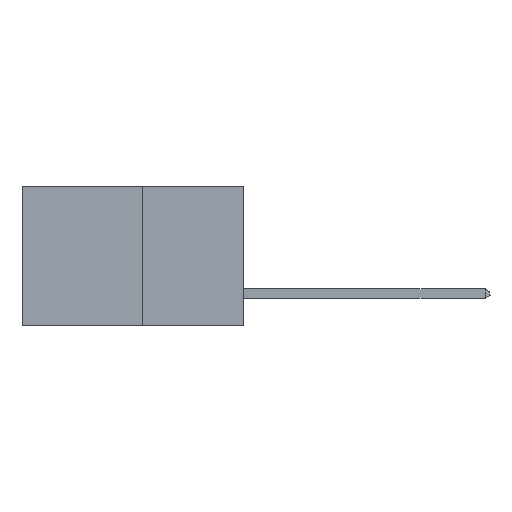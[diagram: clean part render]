
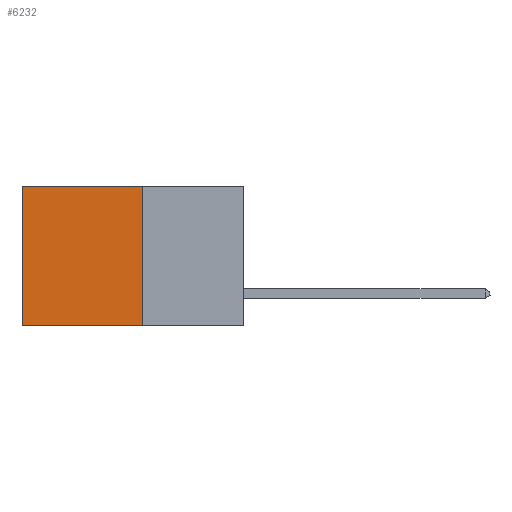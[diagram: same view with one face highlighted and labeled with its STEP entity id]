
A CAD part, left-side view. The second image highlights one B-rep face of the part: STEP entity #6232.
In plain terms, the highlighted planar face has unit normal (-1, 0, 0).
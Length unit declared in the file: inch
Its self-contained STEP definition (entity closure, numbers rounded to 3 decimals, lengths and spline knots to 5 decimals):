
#1770 = CARTESIAN_POINT ( 'NONE',  ( 0.277, 0.59, -0.37 ) ) ;
#2014 = LINE ( 'NONE', #5491, #26398 ) ;
#2191 = CARTESIAN_POINT ( 'NONE',  ( 0.277, 0.27, -0.37 ) ) ;
#2647 = CARTESIAN_POINT ( 'NONE',  ( 0.277, 0.27, 0. ) ) ;
#3800 = DIRECTION ( 'NONE',  ( 0., 0., -1. ) ) ;
#3831 = DIRECTION ( 'NONE',  ( 1., 0., 0. ) ) ;
#3864 = PLANE ( 'NONE',  #15335 ) ;
#4041 = CARTESIAN_POINT ( 'NONE',  ( 0.277, 0.27, -0.37 ) ) ;
#5218 = VERTEX_POINT ( 'NONE', #20524 ) ;
#5420 = DIRECTION ( 'NONE',  ( 0., 1., 0. ) ) ;
#5491 = CARTESIAN_POINT ( 'NONE',  ( 0.277, 0.27, -0.37 ) ) ;
#5721 = EDGE_CURVE ( 'NONE', #5218, #11474, #19144, .T. ) ;
#6232 = ADVANCED_FACE ( 'NONE', ( #10727 ), #3864, .F. ) ;
#6437 = ORIENTED_EDGE ( 'NONE', *, *, #17320, .F. ) ;
#8575 = ORIENTED_EDGE ( 'NONE', *, *, #15449, .F. ) ;
#10727 = FACE_OUTER_BOUND ( 'NONE', #22139, .T. ) ;
#10735 = VECTOR ( 'NONE', #5420, 39.37008 ) ;
#10989 = ORIENTED_EDGE ( 'NONE', *, *, #5721, .T. ) ;
#11474 = VERTEX_POINT ( 'NONE', #1770 ) ;
#12495 = CARTESIAN_POINT ( 'NONE',  ( 0.277, 0.27, 0. ) ) ;
#12855 = DIRECTION ( 'NONE',  ( 0., 0., -1. ) ) ;
#12953 = VECTOR ( 'NONE', #12855, 39.37008 ) ;
#13092 = CARTESIAN_POINT ( 'NONE',  ( 0.277, 0.59, -0.37 ) ) ;
#14027 = VECTOR ( 'NONE', #27221, 39.37008 ) ;
#15335 = AXIS2_PLACEMENT_3D ( 'NONE', #4041, #3831, #3800 ) ;
#15449 = EDGE_CURVE ( 'NONE', #19071, #11474, #20246, .T. ) ;
#16819 = EDGE_CURVE ( 'NONE', #20402, #5218, #16930, .T. ) ;
#16930 = LINE ( 'NONE', #12495, #10735 ) ;
#17320 = EDGE_CURVE ( 'NONE', #20402, #19071, #2014, .T. ) ;
#17822 = CARTESIAN_POINT ( 'NONE',  ( 0.277, 0.27, -0.37 ) ) ;
#19071 = VERTEX_POINT ( 'NONE', #2191 ) ;
#19144 = LINE ( 'NONE', #13092, #12953 ) ;
#20246 = LINE ( 'NONE', #17822, #14027 ) ;
#20402 = VERTEX_POINT ( 'NONE', #2647 ) ;
#20524 = CARTESIAN_POINT ( 'NONE',  ( 0.277, 0.59, 0. ) ) ;
#21968 = DIRECTION ( 'NONE',  ( 0., 0., -1. ) ) ;
#22139 = EDGE_LOOP ( 'NONE', ( #10989, #8575, #6437, #22772 ) ) ;
#22772 = ORIENTED_EDGE ( 'NONE', *, *, #16819, .T. ) ;
#26398 = VECTOR ( 'NONE', #21968, 39.37008 ) ;
#27221 = DIRECTION ( 'NONE',  ( 0., 1., 0. ) ) ;
